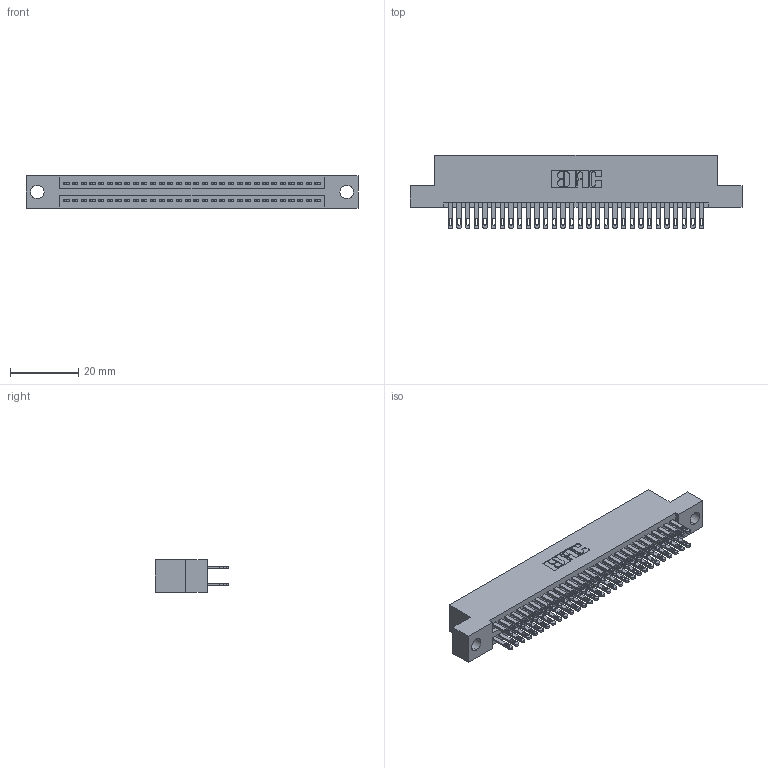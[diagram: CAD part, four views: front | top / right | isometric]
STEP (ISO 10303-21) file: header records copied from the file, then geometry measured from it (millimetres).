
FILE_DESCRIPTION (( 'STEP AP203' ), '1' );
FILE_NAME ('345-060-500-204.STEP', '2021-05-20T05:23:22', ( '' ), ( '' ), 'SwSTEP 2.0', 'SolidWorks 2020', '' );
FILE_SCHEMA (( 'CONFIG_CONTROL_DESIGN' ));
Length unit declared in the file: inch
Products named in the file (3): 345-060-500-204; 345 Part_Flush Mounting Lugs - 0.156 Dia-TI; 345-292-001_345-293-100
Assembly tree (61 placements, depth 2):
  345-060-500-204
    345 Part_Flush Mounting Lugs - 0.156 Dia-TI
    345-292-001_345-293-100  x60
Bounding box: 97.41 x 21.51 x 9.4 mm (x, y, z)
Volume: 9428.4 mm3; surface area: 14167.9 mm2
Topology: 61 solids, 61 shells, 2900 faces, 8837 edges, 5890 vertices
Faces by surface type: plane 1714, cylinder 1186
Entity records: 25503 total; most frequent: CARTESIAN_POINT 4290, ORIENTED_EDGE 4222, DIRECTION 3799, EDGE_CURVE 2111, VECTOR 1855, LINE 1855, VERTEX_POINT 1406, AXIS2_PLACEMENT_3D 972
